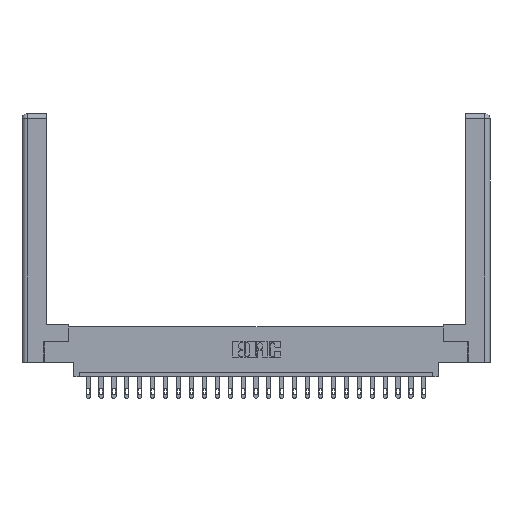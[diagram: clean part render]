
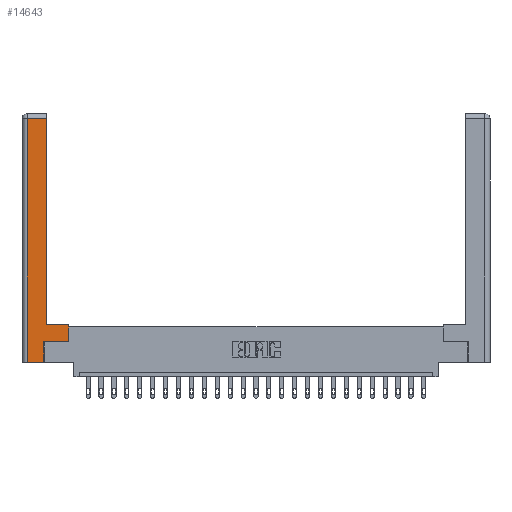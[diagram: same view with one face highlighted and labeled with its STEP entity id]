
A CAD part, top view. The second image highlights one B-rep face of the part: STEP entity #14643.
In plain terms, the highlighted planar face has unit normal (0, 0, 1).
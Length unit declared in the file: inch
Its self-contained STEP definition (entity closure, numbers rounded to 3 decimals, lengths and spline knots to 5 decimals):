
#134 = VECTOR ( 'NONE', #12294, 39.37008 ) ;
#206 = DIRECTION ( 'NONE',  ( 0., 0., -1. ) ) ;
#1003 = CARTESIAN_POINT ( 'NONE',  ( 0.565, 0.45, 0. ) ) ;
#1160 = VECTOR ( 'NONE', #24203, 39.37008 ) ;
#1716 = DIRECTION ( 'NONE',  ( 1., 0., 0. ) ) ;
#1745 = VECTOR ( 'NONE', #21424, 39.37008 ) ;
#2254 = LINE ( 'NONE', #22441, #11852 ) ;
#2492 = EDGE_CURVE ( 'NONE', #2528, #13000, #22646, .T. ) ;
#2528 = VERTEX_POINT ( 'NONE', #6985 ) ;
#3253 = CARTESIAN_POINT ( 'NONE',  ( 0.295, 2.94, 0. ) ) ;
#3403 = CARTESIAN_POINT ( 'NONE',  ( 0.295, 0.45, 0. ) ) ;
#3647 = LINE ( 'NONE', #21067, #4830 ) ;
#3841 = VERTEX_POINT ( 'NONE', #20831 ) ;
#3985 = VERTEX_POINT ( 'NONE', #23153 ) ;
#4830 = VECTOR ( 'NONE', #7764, 39.37008 ) ;
#5010 = LINE ( 'NONE', #24566, #14328 ) ;
#5788 = LINE ( 'NONE', #1003, #134 ) ;
#5906 = VERTEX_POINT ( 'NONE', #18041 ) ;
#6985 = CARTESIAN_POINT ( 'NONE',  ( 0.295, 0.45, 0. ) ) ;
#7330 = LINE ( 'NONE', #16633, #23783 ) ;
#7343 = ORIENTED_EDGE ( 'NONE', *, *, #20508, .T. ) ;
#7372 = EDGE_CURVE ( 'NONE', #13000, #7995, #22336, .T. ) ;
#7764 = DIRECTION ( 'NONE',  ( 0., 1., 0. ) ) ;
#7960 = EDGE_CURVE ( 'NONE', #16250, #14861, #7330, .T. ) ;
#7995 = VERTEX_POINT ( 'NONE', #11366 ) ;
#8040 = AXIS2_PLACEMENT_3D ( 'NONE', #19156, #206, #11724 ) ;
#8717 = DIRECTION ( 'NONE',  ( 0., 1., 0. ) ) ;
#9334 = EDGE_CURVE ( 'NONE', #14861, #3841, #5788, .T. ) ;
#10482 = CARTESIAN_POINT ( 'NONE',  ( 0.295, 3., 0. ) ) ;
#10577 = ORIENTED_EDGE ( 'NONE', *, *, #9334, .T. ) ;
#11002 = DIRECTION ( 'NONE',  ( 0., -1., 0. ) ) ;
#11021 = DIRECTION ( 'NONE',  ( 1., 0., 0. ) ) ;
#11366 = CARTESIAN_POINT ( 'NONE',  ( 0.0615, 2.94, 0. ) ) ;
#11599 = EDGE_CURVE ( 'NONE', #7995, #5906, #2254, .T. ) ;
#11724 = DIRECTION ( 'NONE',  ( -1., 0., 0. ) ) ;
#11769 = ORIENTED_EDGE ( 'NONE', *, *, #2492, .T. ) ;
#11852 = VECTOR ( 'NONE', #11002, 39.37008 ) ;
#11886 = PLANE ( 'NONE',  #8040 ) ;
#12084 = ORIENTED_EDGE ( 'NONE', *, *, #7960, .T. ) ;
#12294 = DIRECTION ( 'NONE',  ( 0., 1., 0. ) ) ;
#12510 = VECTOR ( 'NONE', #8717, 39.37008 ) ;
#13000 = VERTEX_POINT ( 'NONE', #3253 ) ;
#13364 = ORIENTED_EDGE ( 'NONE', *, *, #11599, .T. ) ;
#14328 = VECTOR ( 'NONE', #1716, 39.37008 ) ;
#14643 = ADVANCED_FACE ( 'NONE', ( #15293 ), #11886, .F. ) ;
#14861 = VERTEX_POINT ( 'NONE', #17901 ) ;
#15293 = FACE_OUTER_BOUND ( 'NONE', #15722, .T. ) ;
#15681 = CARTESIAN_POINT ( 'NONE',  ( 0.0615, 2.94, 0. ) ) ;
#15722 = EDGE_LOOP ( 'NONE', ( #11769, #17803, #13364, #23492, #7343, #12084, #10577, #21461 ) ) ;
#16250 = VERTEX_POINT ( 'NONE', #23730 ) ;
#16633 = CARTESIAN_POINT ( 'NONE',  ( 0.565, 0.245, 0. ) ) ;
#17803 = ORIENTED_EDGE ( 'NONE', *, *, #7372, .T. ) ;
#17901 = CARTESIAN_POINT ( 'NONE',  ( 0.565, 0.245, 0. ) ) ;
#18041 = CARTESIAN_POINT ( 'NONE',  ( 0.0615, 0., 0. ) ) ;
#19156 = CARTESIAN_POINT ( 'NONE',  ( 0., 0., 0. ) ) ;
#20508 = EDGE_CURVE ( 'NONE', #3985, #16250, #3647, .T. ) ;
#20831 = CARTESIAN_POINT ( 'NONE',  ( 0.565, 0.45, 0. ) ) ;
#21067 = CARTESIAN_POINT ( 'NONE',  ( 0.265, 0.245, 0. ) ) ;
#21424 = DIRECTION ( 'NONE',  ( -1., 0., 0. ) ) ;
#21461 = ORIENTED_EDGE ( 'NONE', *, *, #22754, .T. ) ;
#22336 = LINE ( 'NONE', #15681, #1745 ) ;
#22441 = CARTESIAN_POINT ( 'NONE',  ( 0.0615, 0., 0. ) ) ;
#22646 = LINE ( 'NONE', #10482, #12510 ) ;
#22754 = EDGE_CURVE ( 'NONE', #3841, #2528, #24444, .T. ) ;
#23153 = CARTESIAN_POINT ( 'NONE',  ( 0.265, 0., 0. ) ) ;
#23492 = ORIENTED_EDGE ( 'NONE', *, *, #24169, .T. ) ;
#23730 = CARTESIAN_POINT ( 'NONE',  ( 0.265, 0.245, 0. ) ) ;
#23783 = VECTOR ( 'NONE', #11021, 39.37008 ) ;
#24169 = EDGE_CURVE ( 'NONE', #5906, #3985, #5010, .T. ) ;
#24203 = DIRECTION ( 'NONE',  ( -1., 0., 0. ) ) ;
#24444 = LINE ( 'NONE', #3403, #1160 ) ;
#24566 = CARTESIAN_POINT ( 'NONE',  ( 0.265, 0., 0. ) ) ;
